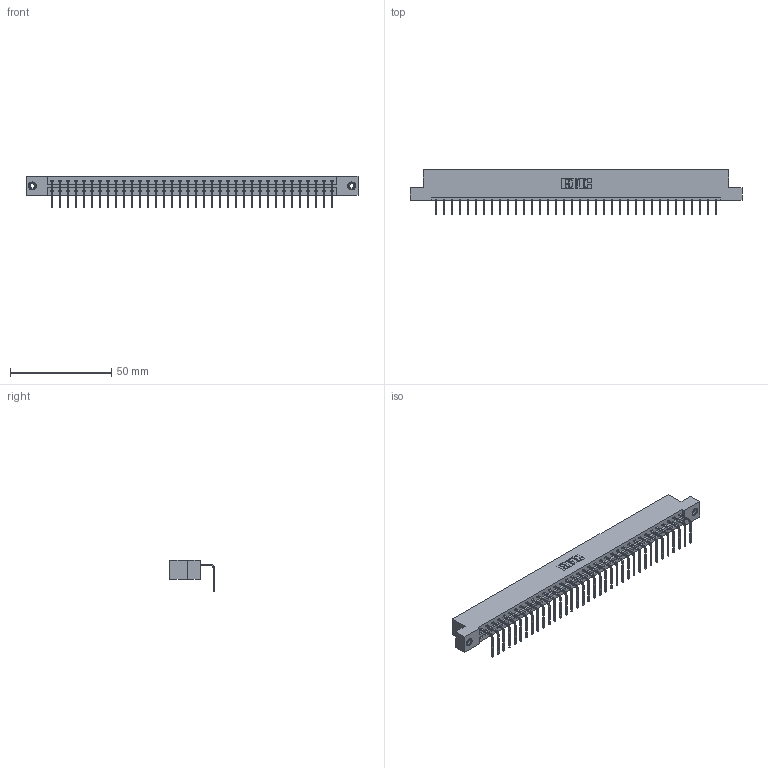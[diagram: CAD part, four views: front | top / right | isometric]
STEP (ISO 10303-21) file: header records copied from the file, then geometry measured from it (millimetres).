
FILE_DESCRIPTION (( 'STEP AP203' ), '1' );
FILE_NAME ('333-036-558-108.STEP', '2018-08-03T01:42:36', ( '' ), ( '' ), 'SwSTEP 2.0', 'SolidWorks 2016', '' );
FILE_SCHEMA (( 'CONFIG_CONTROL_DESIGN' ));
Length unit declared in the file: inch
Products named in the file (4): 345-292-001_558 Tail - 2; 345-250-001_345-250-003-102; 333-036-558-108; 333 Part_Flush - .156 Dia - TI
Assembly tree (39 placements, depth 2):
  333-036-558-108
    333 Part_Flush - .156 Dia - TI
    345-292-001_558 Tail - 2  x36
    345-250-001_345-250-003-102  x2
Bounding box: 164.19 x 22.17 x 15.37 mm (x, y, z)
Volume: 16583.5 mm3; surface area: 18665.2 mm2
Topology: 39 solids, 39 shells, 2334 faces, 6999 edges, 4610 vertices
Faces by surface type: plane 1686, cylinder 632, cone 12, torus 4
Entity records: 24054 total; most frequent: CARTESIAN_POINT 4133, ORIENTED_EDGE 4098, DIRECTION 3531, EDGE_CURVE 2049, LINE 1901, VECTOR 1901, VERTEX_POINT 1360, AXIS2_PLACEMENT_3D 815
